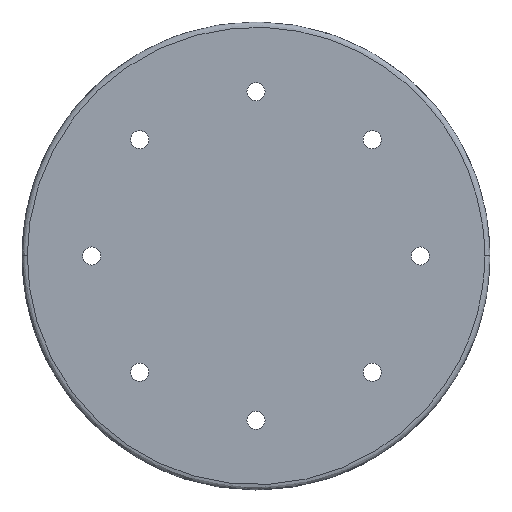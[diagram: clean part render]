
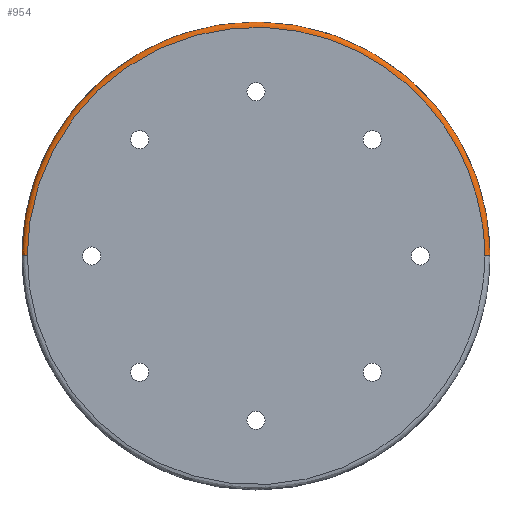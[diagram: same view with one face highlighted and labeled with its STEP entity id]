
A CAD part, top view. The second image highlights one B-rep face of the part: STEP entity #954.
In plain terms, the highlighted free-form (B-spline) face has degree [3, 3] with [4, 4] control points.
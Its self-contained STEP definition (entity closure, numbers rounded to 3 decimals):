
#141 = CARTESIAN_POINT ( 'NONE',  ( -22., 0., 1.093 ) ) ;
#143 = CARTESIAN_POINT ( 'NONE',  ( 22.032, 0., 1.09 ) ) ;
#175 = CARTESIAN_POINT ( 'NONE',  ( -22., 0., 0.8 ) ) ;
#473 = EDGE_CURVE ( 'NONE', #8456, #4229, #2569, .T. ) ;
#772 = ORIENTED_EDGE ( 'NONE', *, *, #6226, .F. ) ;
#820 = EDGE_CURVE ( 'NONE', #1847, #4229, #9482, .T. ) ;
#870 = CARTESIAN_POINT ( 'NONE',  ( -22.032, 44.063, 1.09 ) ) ;
#954 = ADVANCED_FACE ( 'NONE', ( #6413 ), #1886, .T. ) ;
#1007 = CARTESIAN_POINT ( 'NONE',  ( 21.5, 43., 1.3 ) ) ;
#1183 = CARTESIAN_POINT ( 'NONE',  ( 22., 0., 0.8 ) ) ;
#1188 = CARTESIAN_POINT ( 'NONE',  ( 22., 0., 1.093 ) ) ;
#1444 = EDGE_CURVE ( 'NONE', #8456, #2294, #3819, .T. ) ;
#1559 = CARTESIAN_POINT ( 'NONE',  ( 21.45, 42.9, 1.298 ) ) ;
#1589 = ORIENTED_EDGE ( 'NONE', *, *, #1444, .T. ) ;
#1596 = CARTESIAN_POINT ( 'NONE',  ( 21.998, 0., 0.75 ) ) ;
#1638 = CARTESIAN_POINT ( 'NONE',  ( -22., 0., 0.8 ) ) ;
#1756 = ORIENTED_EDGE ( 'NONE', *, *, #820, .T. ) ;
#1847 = VERTEX_POINT ( 'NONE', #1183 ) ;
#1886 =( BOUNDED_SURFACE ( )  B_SPLINE_SURFACE ( 3, 3, ( 
 ( #5197, #1559, #7417, #3005 ),
 ( #8171, #3751, #8898, #4488 ),
 ( #143, #5229, #870, #5975 ),
 ( #1596, #6714, #2331, #7461 ) ),
 .UNSPECIFIED., .F., .F., .T. ) 
 B_SPLINE_SURFACE_WITH_KNOTS ( ( 4, 4 ),
 ( 4, 4 ),
 ( 0., 1. ),
 ( 0., 1. ),
 .UNSPECIFIED. ) 
 GEOMETRIC_REPRESENTATION_ITEM ( )  RATIONAL_B_SPLINE_SURFACE ( (
 ( 1., 0.333, 0.333, 1.),
 ( 0.755, 0.252, 0.252, 0.755),
 ( 0.755, 0.252, 0.252, 0.755),
 ( 1., 0.333, 0.333, 1.) ) ) 
 REPRESENTATION_ITEM ( '' )  SURFACE ( )  );
#2294 = VERTEX_POINT ( 'NONE', #2902 ) ;
#2331 = CARTESIAN_POINT ( 'NONE',  ( -21.998, 43.995, 0.75 ) ) ;
#2569 =( BOUNDED_CURVE ( )  B_SPLINE_CURVE ( 3, ( #4516, #6713, #141, #175 ),
 .UNSPECIFIED., .F., .T. ) 
 B_SPLINE_CURVE_WITH_KNOTS ( ( 4, 4 ),
 ( 0.063, 0.937 ),
 .UNSPECIFIED. ) 
 CURVE ( )  GEOMETRIC_REPRESENTATION_ITEM ( )  RATIONAL_B_SPLINE_CURVE ( ( 0.957, 0.77, 0.77, 0.957 ) ) 
 REPRESENTATION_ITEM ( '' )  );
#2632 = CARTESIAN_POINT ( 'NONE',  ( 21.5, 0., 1.3 ) ) ;
#2902 = CARTESIAN_POINT ( 'NONE',  ( 21.5, 0., 1.3 ) ) ;
#2935 =( BOUNDED_CURVE ( )  B_SPLINE_CURVE ( 3, ( #6295, #1188, #7041, #2632 ),
 .UNSPECIFIED., .F., .F. ) 
 B_SPLINE_CURVE_WITH_KNOTS ( ( 4, 4 ),
 ( 0.063, 0.937 ),
 .UNSPECIFIED. ) 
 CURVE ( )  GEOMETRIC_REPRESENTATION_ITEM ( )  RATIONAL_B_SPLINE_CURVE ( ( 0.957, 0.77, 0.77, 0.957 ) ) 
 REPRESENTATION_ITEM ( '' )  );
#3005 = CARTESIAN_POINT ( 'NONE',  ( -21.45, 0., 1.298 ) ) ;
#3143 = CARTESIAN_POINT ( 'NONE',  ( -21.5, 0., 1.3 ) ) ;
#3688 = CARTESIAN_POINT ( 'NONE',  ( 0., 0., 0.8 ) ) ;
#3751 = CARTESIAN_POINT ( 'NONE',  ( 21.79, 43.58, 1.332 ) ) ;
#3819 =( BOUNDED_CURVE ( )  B_SPLINE_CURVE ( 3, ( #3143, #3896, #1007, #6119 ),
 .UNSPECIFIED., .F., .T. ) 
 B_SPLINE_CURVE_WITH_KNOTS ( ( 4, 4 ),
 ( 0., 1. ),
 .UNSPECIFIED. ) 
 CURVE ( )  GEOMETRIC_REPRESENTATION_ITEM ( )  RATIONAL_B_SPLINE_CURVE ( ( 0.957, 0.319, 0.319, 0.957 ) ) 
 REPRESENTATION_ITEM ( '' )  );
#3896 = CARTESIAN_POINT ( 'NONE',  ( -21.5, 43., 1.3 ) ) ;
#4229 = VERTEX_POINT ( 'NONE', #1638 ) ;
#4421 = DIRECTION ( 'NONE',  ( 1., 0., 0. ) ) ;
#4488 = CARTESIAN_POINT ( 'NONE',  ( -21.79, 0., 1.332 ) ) ;
#4516 = CARTESIAN_POINT ( 'NONE',  ( -21.5, 0., 1.3 ) ) ;
#4820 = AXIS2_PLACEMENT_3D ( 'NONE', #3688, #8844, #4421 ) ;
#5197 = CARTESIAN_POINT ( 'NONE',  ( 21.45, 0., 1.298 ) ) ;
#5229 = CARTESIAN_POINT ( 'NONE',  ( 22.032, 44.063, 1.09 ) ) ;
#5846 = EDGE_LOOP ( 'NONE', ( #1589, #772, #1756, #8256 ) ) ;
#5874 = CARTESIAN_POINT ( 'NONE',  ( -21.5, 0., 1.3 ) ) ;
#5975 = CARTESIAN_POINT ( 'NONE',  ( -22.032, 0., 1.09 ) ) ;
#6119 = CARTESIAN_POINT ( 'NONE',  ( 21.5, 0., 1.3 ) ) ;
#6226 = EDGE_CURVE ( 'NONE', #1847, #2294, #2935, .T. ) ;
#6295 = CARTESIAN_POINT ( 'NONE',  ( 22., 0., 0.8 ) ) ;
#6413 = FACE_OUTER_BOUND ( 'NONE', #5846, .T. ) ;
#6713 = CARTESIAN_POINT ( 'NONE',  ( -21.793, 0., 1.3 ) ) ;
#6714 = CARTESIAN_POINT ( 'NONE',  ( 21.998, 43.995, 0.75 ) ) ;
#7041 = CARTESIAN_POINT ( 'NONE',  ( 21.793, 0., 1.3 ) ) ;
#7417 = CARTESIAN_POINT ( 'NONE',  ( -21.45, 42.9, 1.298 ) ) ;
#7461 = CARTESIAN_POINT ( 'NONE',  ( -21.998, 0., 0.75 ) ) ;
#8171 = CARTESIAN_POINT ( 'NONE',  ( 21.79, 0., 1.332 ) ) ;
#8256 = ORIENTED_EDGE ( 'NONE', *, *, #473, .F. ) ;
#8456 = VERTEX_POINT ( 'NONE', #5874 ) ;
#8844 = DIRECTION ( 'NONE',  ( 0., 0., 1. ) ) ;
#8898 = CARTESIAN_POINT ( 'NONE',  ( -21.79, 43.58, 1.332 ) ) ;
#9482 = CIRCLE ( 'NONE', #4820, 22. ) ;
